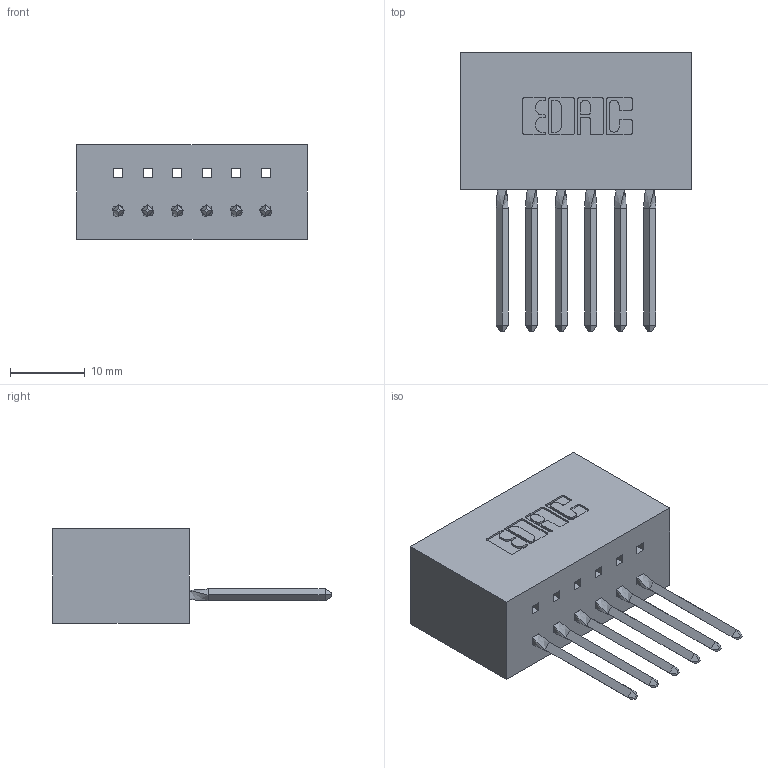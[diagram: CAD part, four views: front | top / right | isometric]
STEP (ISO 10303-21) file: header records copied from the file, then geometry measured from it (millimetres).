
FILE_DESCRIPTION (( 'STEP AP203' ), '1' );
FILE_NAME ('317-006-542-601.STEP', '2020-02-27T12:36:57', ( '' ), ( '' ), 'SwSTEP 2.0', 'SolidWorks 2016', '' );
FILE_SCHEMA (( 'CONFIG_CONTROL_DESIGN' ));
Length unit declared in the file: inch
Products named in the file (3): 317-006-542-601; 317-290-003_542; 317 Part_Lugless
Assembly tree (7 placements, depth 2):
  317-006-542-601
    317 Part_Lugless
    317-290-003_542  x6
Bounding box: 30.99 x 37.34 x 12.7 mm (x, y, z)
Volume: 5416.2 mm3; surface area: 5841.1 mm2
Topology: 7 solids, 7 shells, 540 faces, 1541 edges, 998 vertices
Faces by surface type: plane 434, cylinder 82, bspline 24
Entity records: 12111 total; most frequent: CARTESIAN_POINT 2383, ORIENTED_EDGE 2052, DIRECTION 1770, EDGE_CURVE 1026, VECTOR 864, LINE 864, VERTEX_POINT 678, AXIS2_PLACEMENT_3D 453
